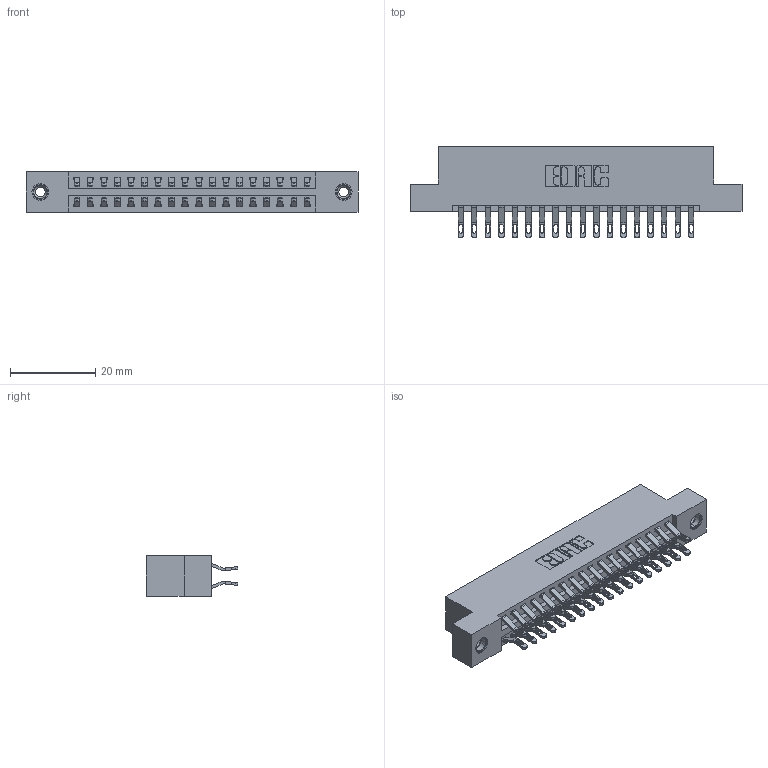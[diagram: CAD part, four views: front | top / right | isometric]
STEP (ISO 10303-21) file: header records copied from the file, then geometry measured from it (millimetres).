
FILE_DESCRIPTION (( 'STEP AP203' ), '1' );
FILE_NAME ('396-036-555-208.STEP', '2019-10-30T07:41:21', ( '' ), ( '' ), 'SwSTEP 2.0', 'SolidWorks 2016', '' );
FILE_SCHEMA (( 'CONFIG_CONTROL_DESIGN' ));
Length unit declared in the file: inch
Products named in the file (4): 345-250-001_345-250-003-102; 345-292-001_555 Tail; 396-036-555-208; 346 Part_Flush Mounting Lugs - 0.156 Dia-TI
Assembly tree (39 placements, depth 2):
  396-036-555-208
    346 Part_Flush Mounting Lugs - 0.156 Dia-TI
    345-292-001_555 Tail  x36
    345-250-001_345-250-003-102  x2
Bounding box: 77.72 x 21.46 x 9.4 mm (x, y, z)
Volume: 7490.6 mm3; surface area: 10311.3 mm2
Topology: 39 solids, 39 shells, 2270 faces, 7053 edges, 4694 vertices
Faces by surface type: plane 1296, cylinder 958, cone 12, torus 4
Entity records: 16490 total; most frequent: CARTESIAN_POINT 2769, ORIENTED_EDGE 2666, DIRECTION 2487, EDGE_CURVE 1333, LINE 1089, VECTOR 1089, VERTEX_POINT 884, AXIS2_PLACEMENT_3D 699
